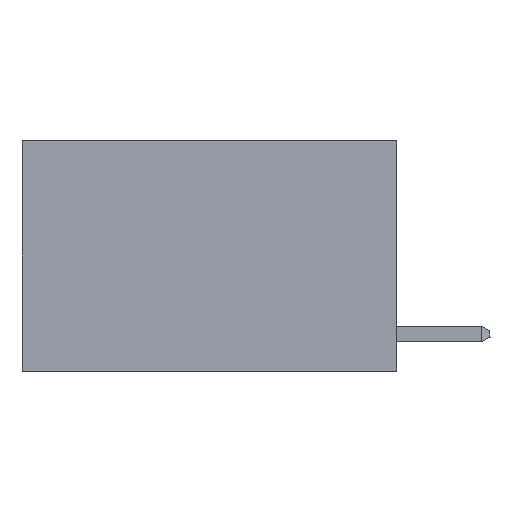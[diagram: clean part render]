
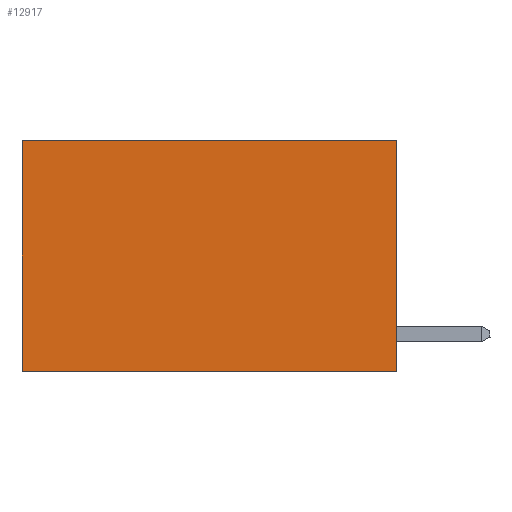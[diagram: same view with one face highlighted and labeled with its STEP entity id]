
A CAD part, left-side view. The second image highlights one B-rep face of the part: STEP entity #12917.
In plain terms, the highlighted planar face has unit normal (-1, 0, 0).
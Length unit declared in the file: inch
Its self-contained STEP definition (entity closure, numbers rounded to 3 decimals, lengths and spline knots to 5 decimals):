
#46 = FACE_OUTER_BOUND ( 'NONE', #14147, .T. ) ;
#96 = DIRECTION ( 'NONE',  ( 0., 1., 0. ) ) ;
#618 = ORIENTED_EDGE ( 'NONE', *, *, #12042, .T. ) ;
#763 = ORIENTED_EDGE ( 'NONE', *, *, #26243, .F. ) ;
#2552 = CARTESIAN_POINT ( 'NONE',  ( 0.2625, 0., 0. ) ) ;
#2746 = VECTOR ( 'NONE', #26981, 39.37008 ) ;
#3569 = CARTESIAN_POINT ( 'NONE',  ( 0.2625, 0., 0. ) ) ;
#5942 = ORIENTED_EDGE ( 'NONE', *, *, #26940, .F. ) ;
#6004 = CARTESIAN_POINT ( 'NONE',  ( 0.2625, 0., -0.37 ) ) ;
#6022 = CARTESIAN_POINT ( 'NONE',  ( 0.2625, 0.6, 0. ) ) ;
#6900 = CARTESIAN_POINT ( 'NONE',  ( 0.2625, 0.6, 0. ) ) ;
#7187 = CARTESIAN_POINT ( 'NONE',  ( 0.2625, 0., -0.37 ) ) ;
#7466 = DIRECTION ( 'NONE',  ( 1., 0., 0. ) ) ;
#9057 = LINE ( 'NONE', #3569, #19658 ) ;
#9597 = VECTOR ( 'NONE', #25496, 39.37008 ) ;
#9604 = ORIENTED_EDGE ( 'NONE', *, *, #24848, .T. ) ;
#10523 = VERTEX_POINT ( 'NONE', #7187 ) ;
#11499 = AXIS2_PLACEMENT_3D ( 'NONE', #20130, #7466, #22264 ) ;
#12042 = EDGE_CURVE ( 'NONE', #13313, #16361, #18269, .T. ) ;
#12917 = ADVANCED_FACE ( 'NONE', ( #46 ), #26337, .F. ) ;
#13313 = VERTEX_POINT ( 'NONE', #6900 ) ;
#14147 = EDGE_LOOP ( 'NONE', ( #618, #763, #5942, #9604 ) ) ;
#15227 = VERTEX_POINT ( 'NONE', #2552 ) ;
#16209 = DIRECTION ( 'NONE',  ( 0., 1., 0. ) ) ;
#16361 = VERTEX_POINT ( 'NONE', #19989 ) ;
#18269 = LINE ( 'NONE', #6022, #2746 ) ;
#19658 = VECTOR ( 'NONE', #16209, 39.37008 ) ;
#19989 = CARTESIAN_POINT ( 'NONE',  ( 0.2625, 0.6, -0.37 ) ) ;
#20130 = CARTESIAN_POINT ( 'NONE',  ( 0.2625, 0., 0. ) ) ;
#21322 = CARTESIAN_POINT ( 'NONE',  ( 0.2625, 0., 0. ) ) ;
#21534 = LINE ( 'NONE', #21322, #9597 ) ;
#21901 = LINE ( 'NONE', #6004, #26748 ) ;
#22264 = DIRECTION ( 'NONE',  ( 0., 0., -1. ) ) ;
#24848 = EDGE_CURVE ( 'NONE', #15227, #13313, #9057, .T. ) ;
#25496 = DIRECTION ( 'NONE',  ( 0., 0., -1. ) ) ;
#26243 = EDGE_CURVE ( 'NONE', #10523, #16361, #21901, .T. ) ;
#26337 = PLANE ( 'NONE',  #11499 ) ;
#26748 = VECTOR ( 'NONE', #96, 39.37008 ) ;
#26940 = EDGE_CURVE ( 'NONE', #15227, #10523, #21534, .T. ) ;
#26981 = DIRECTION ( 'NONE',  ( 0., 0., -1. ) ) ;
